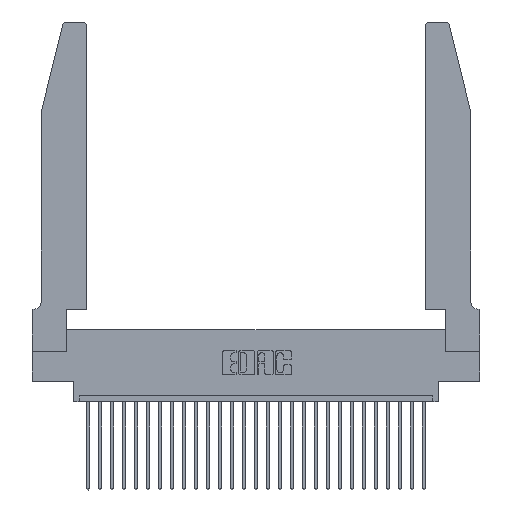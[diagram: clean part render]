
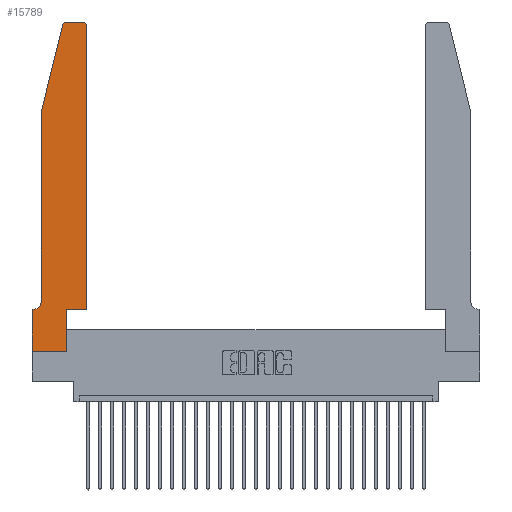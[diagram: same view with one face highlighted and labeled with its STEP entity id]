
A CAD part, top view. The second image highlights one B-rep face of the part: STEP entity #15789.
In plain terms, the highlighted planar face has unit normal (0, 0, 1).
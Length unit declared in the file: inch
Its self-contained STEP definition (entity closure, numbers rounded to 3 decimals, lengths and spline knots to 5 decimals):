
#60 = ORIENTED_EDGE ( 'NONE', *, *, #159, .T. ) ;
#159 = EDGE_CURVE ( 'NONE', #14211, #9356, #9933, .T. ) ;
#343 = VERTEX_POINT ( 'NONE', #19643 ) ;
#527 = VECTOR ( 'NONE', #25018, 39.37008 ) ;
#533 = CARTESIAN_POINT ( 'NONE',  ( 0.4205, 2.72, 0.37 ) ) ;
#692 = ORIENTED_EDGE ( 'NONE', *, *, #19908, .T. ) ;
#1111 = VERTEX_POINT ( 'NONE', #28508 ) ;
#1288 = DIRECTION ( 'NONE',  ( 1., 0., 0. ) ) ;
#1362 = CARTESIAN_POINT ( 'NONE',  ( 0.4505, 0.35, 0.37 ) ) ;
#1607 = LINE ( 'NONE', #1362, #3279 ) ;
#2472 = ORIENTED_EDGE ( 'NONE', *, *, #9651, .T. ) ;
#3101 = FACE_OUTER_BOUND ( 'NONE', #27921, .T. ) ;
#3279 = VECTOR ( 'NONE', #3536, 39.37008 ) ;
#3476 = CARTESIAN_POINT ( 'NONE',  ( 0., 0.35, 0.37 ) ) ;
#3495 = CARTESIAN_POINT ( 'NONE',  ( 0.0755, 2., 0.37 ) ) ;
#3536 = DIRECTION ( 'NONE',  ( 0., 1., 0. ) ) ;
#4212 = CARTESIAN_POINT ( 'NONE',  ( 0.0755, 0.42, 0.37 ) ) ;
#4334 = LINE ( 'NONE', #8835, #27030 ) ;
#4914 = DIRECTION ( 'NONE',  ( 0., 1., 0. ) ) ;
#5232 = VERTEX_POINT ( 'NONE', #3495 ) ;
#5487 = VECTOR ( 'NONE', #4914, 39.37008 ) ;
#5525 = VECTOR ( 'NONE', #20050, 39.37008 ) ;
#5538 = AXIS2_PLACEMENT_3D ( 'NONE', #533, #15820, #24915 ) ;
#5829 = CARTESIAN_POINT ( 'NONE',  ( 0.0055, 0.35, 0.37 ) ) ;
#6103 = CIRCLE ( 'NONE', #23473, 0.07 ) ;
#6519 = VERTEX_POINT ( 'NONE', #13671 ) ;
#7257 = CARTESIAN_POINT ( 'NONE',  ( 0.0055, 0.42, 0.37 ) ) ;
#7717 = AXIS2_PLACEMENT_3D ( 'NONE', #25777, #12387, #16679 ) ;
#7843 = DIRECTION ( 'NONE',  ( 0., -1., 0. ) ) ;
#8002 = ORIENTED_EDGE ( 'NONE', *, *, #25364, .T. ) ;
#8451 = AXIS2_PLACEMENT_3D ( 'NONE', #3476, #18515, #1288 ) ;
#8458 = VERTEX_POINT ( 'NONE', #18560 ) ;
#8705 = ORIENTED_EDGE ( 'NONE', *, *, #25272, .T. ) ;
#8835 = CARTESIAN_POINT ( 'NONE',  ( 0.2605, 2.75, 0.37 ) ) ;
#8867 = CARTESIAN_POINT ( 'NONE',  ( 0.4205, 2.75, 0.37 ) ) ;
#9356 = VERTEX_POINT ( 'NONE', #19963 ) ;
#9541 = EDGE_CURVE ( 'NONE', #9356, #343, #21074, .T. ) ;
#9651 = EDGE_CURVE ( 'NONE', #5232, #15477, #28356, .T. ) ;
#9690 = PLANE ( 'NONE',  #8451 ) ;
#9933 = LINE ( 'NONE', #12258, #14374 ) ;
#10901 = DIRECTION ( 'NONE',  ( -1., 0., 0. ) ) ;
#11940 = EDGE_CURVE ( 'NONE', #8458, #6519, #1607, .T. ) ;
#12182 = CARTESIAN_POINT ( 'NONE',  ( 0.25487, 2.72718, 0.37 ) ) ;
#12249 = DIRECTION ( 'NONE',  ( -1., 0., 0. ) ) ;
#12258 = CARTESIAN_POINT ( 'NONE',  ( 0., 0., 0.37 ) ) ;
#12387 = DIRECTION ( 'NONE',  ( 0., 0., 1. ) ) ;
#12795 = ORIENTED_EDGE ( 'NONE', *, *, #21394, .T. ) ;
#13626 = VECTOR ( 'NONE', #10901, 39.37008 ) ;
#13671 = CARTESIAN_POINT ( 'NONE',  ( 0.4505, 2.72, 0.37 ) ) ;
#14099 = LINE ( 'NONE', #26839, #5525 ) ;
#14211 = VERTEX_POINT ( 'NONE', #20839 ) ;
#14306 = CARTESIAN_POINT ( 'NONE',  ( 0.0755, 2., 0.37 ) ) ;
#14374 = VECTOR ( 'NONE', #7843, 39.37008 ) ;
#15130 = VERTEX_POINT ( 'NONE', #17999 ) ;
#15207 = VECTOR ( 'NONE', #19787, 39.37008 ) ;
#15477 = VERTEX_POINT ( 'NONE', #4212 ) ;
#15624 = CARTESIAN_POINT ( 'NONE',  ( 0., 0., 0.37 ) ) ;
#15703 = VERTEX_POINT ( 'NONE', #12182 ) ;
#15789 = ADVANCED_FACE ( 'NONE', ( #3101 ), #9690, .T. ) ;
#15820 = DIRECTION ( 'NONE',  ( 0., 0., 1. ) ) ;
#16367 = DIRECTION ( 'NONE',  ( 0., 0., -1. ) ) ;
#16679 = DIRECTION ( 'NONE',  ( 1., 0., 0. ) ) ;
#16819 = VERTEX_POINT ( 'NONE', #5829 ) ;
#16937 = ORIENTED_EDGE ( 'NONE', *, *, #11940, .T. ) ;
#17519 = CARTESIAN_POINT ( 'NONE',  ( 0.0755, 0.35, 0.37 ) ) ;
#17838 = CIRCLE ( 'NONE', #5538, 0.03 ) ;
#17999 = CARTESIAN_POINT ( 'NONE',  ( 0.2865, 0.35, 0.37 ) ) ;
#18026 = DIRECTION ( 'NONE',  ( 0., -1., 0. ) ) ;
#18515 = DIRECTION ( 'NONE',  ( 0., 0., 1. ) ) ;
#18560 = CARTESIAN_POINT ( 'NONE',  ( 0.4505, 0.35, 0.37 ) ) ;
#19643 = CARTESIAN_POINT ( 'NONE',  ( 0.2865, 0., 0.37 ) ) ;
#19787 = DIRECTION ( 'NONE',  ( 1., 0., 0. ) ) ;
#19908 = EDGE_CURVE ( 'NONE', #15703, #5232, #25986, .T. ) ;
#19963 = CARTESIAN_POINT ( 'NONE',  ( 0., 0., 0.37 ) ) ;
#19970 = CARTESIAN_POINT ( 'NONE',  ( 0.2865, 0.35, 0.37 ) ) ;
#20050 = DIRECTION ( 'NONE',  ( 1., 0., 0. ) ) ;
#20839 = CARTESIAN_POINT ( 'NONE',  ( 0., 0.35, 0.37 ) ) ;
#21074 = LINE ( 'NONE', #15624, #15207 ) ;
#21210 = LINE ( 'NONE', #17519, #13626 ) ;
#21394 = EDGE_CURVE ( 'NONE', #15130, #8458, #14099, .T. ) ;
#23017 = LINE ( 'NONE', #19970, #5487 ) ;
#23473 = AXIS2_PLACEMENT_3D ( 'NONE', #7257, #16367, #12249 ) ;
#23727 = EDGE_CURVE ( 'NONE', #1111, #15703, #28187, .T. ) ;
#24855 = VECTOR ( 'NONE', #18026, 39.37008 ) ;
#24915 = DIRECTION ( 'NONE',  ( 1., 0., 0. ) ) ;
#25018 = DIRECTION ( 'NONE',  ( -0.239, -0.971, 0. ) ) ;
#25193 = ORIENTED_EDGE ( 'NONE', *, *, #26502, .T. ) ;
#25272 = EDGE_CURVE ( 'NONE', #343, #15130, #23017, .T. ) ;
#25364 = EDGE_CURVE ( 'NONE', #6519, #27641, #17838, .T. ) ;
#25777 = CARTESIAN_POINT ( 'NONE',  ( 0.284, 2.72, 0.37 ) ) ;
#25986 = LINE ( 'NONE', #27251, #527 ) ;
#26032 = ORIENTED_EDGE ( 'NONE', *, *, #26933, .T. ) ;
#26168 = DIRECTION ( 'NONE',  ( -1., 0., 0. ) ) ;
#26502 = EDGE_CURVE ( 'NONE', #15477, #16819, #6103, .T. ) ;
#26823 = ORIENTED_EDGE ( 'NONE', *, *, #9541, .T. ) ;
#26839 = CARTESIAN_POINT ( 'NONE',  ( 0.4505, 0.35, 0.37 ) ) ;
#26933 = EDGE_CURVE ( 'NONE', #16819, #14211, #21210, .T. ) ;
#27030 = VECTOR ( 'NONE', #26168, 39.37008 ) ;
#27251 = CARTESIAN_POINT ( 'NONE',  ( 0.0755, 2., 0.37 ) ) ;
#27322 = ORIENTED_EDGE ( 'NONE', *, *, #28119, .T. ) ;
#27641 = VERTEX_POINT ( 'NONE', #8867 ) ;
#27809 = ORIENTED_EDGE ( 'NONE', *, *, #23727, .T. ) ;
#27921 = EDGE_LOOP ( 'NONE', ( #27322, #27809, #692, #2472, #25193, #26032, #60, #26823, #8705, #12795, #16937, #8002 ) ) ;
#28119 = EDGE_CURVE ( 'NONE', #27641, #1111, #4334, .T. ) ;
#28187 = CIRCLE ( 'NONE', #7717, 0.03 ) ;
#28356 = LINE ( 'NONE', #14306, #24855 ) ;
#28508 = CARTESIAN_POINT ( 'NONE',  ( 0.284, 2.75, 0.37 ) ) ;
